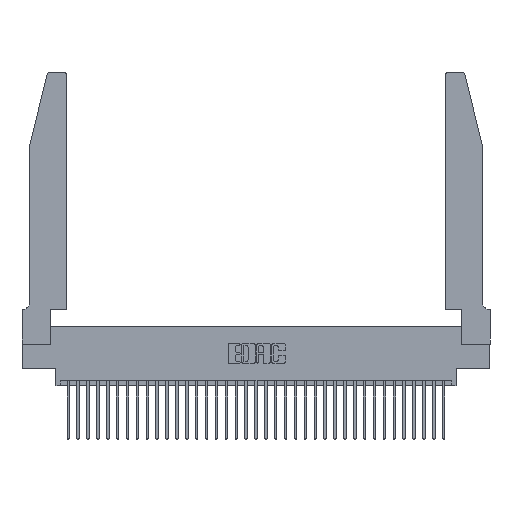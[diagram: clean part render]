
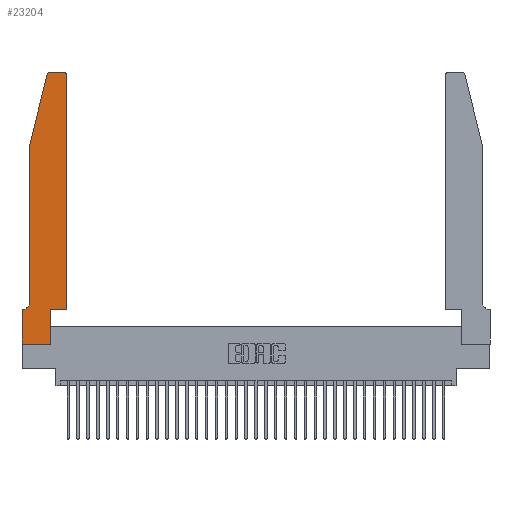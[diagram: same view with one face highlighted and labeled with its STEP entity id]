
A CAD part, top view. The second image highlights one B-rep face of the part: STEP entity #23204.
In plain terms, the highlighted planar face has unit normal (0, 0, 1).
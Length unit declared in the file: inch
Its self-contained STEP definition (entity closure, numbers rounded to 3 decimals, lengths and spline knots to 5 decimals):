
#298 = VECTOR ( 'NONE', #17683, 39.37008 ) ;
#578 = CIRCLE ( 'NONE', #31965, 0.07 ) ;
#1202 = DIRECTION ( 'NONE',  ( 0., 0., -1. ) ) ;
#1288 = VECTOR ( 'NONE', #32360, 39.37008 ) ;
#2203 = CARTESIAN_POINT ( 'NONE',  ( 0.0755, 2., 0.37 ) ) ;
#2274 = ORIENTED_EDGE ( 'NONE', *, *, #16135, .T. ) ;
#2450 = DIRECTION ( 'NONE',  ( -1., 0., 0. ) ) ;
#2820 = LINE ( 'NONE', #4468, #11868 ) ;
#3129 = ORIENTED_EDGE ( 'NONE', *, *, #24336, .T. ) ;
#3599 = CARTESIAN_POINT ( 'NONE',  ( 0., 0.35, 0.37 ) ) ;
#3640 = FACE_OUTER_BOUND ( 'NONE', #35420, .T. ) ;
#3865 = EDGE_CURVE ( 'NONE', #8779, #29767, #17887, .T. ) ;
#4079 = CARTESIAN_POINT ( 'NONE',  ( 0.4205, 2.75, 0.37 ) ) ;
#4468 = CARTESIAN_POINT ( 'NONE',  ( 0.0755, 2., 0.37 ) ) ;
#4948 = CARTESIAN_POINT ( 'NONE',  ( 0., 0., 0.37 ) ) ;
#5295 = ORIENTED_EDGE ( 'NONE', *, *, #23251, .T. ) ;
#5434 = DIRECTION ( 'NONE',  ( 0., -1., 0. ) ) ;
#6022 = CARTESIAN_POINT ( 'NONE',  ( 0., 0., 0.37 ) ) ;
#6300 = CARTESIAN_POINT ( 'NONE',  ( 0.2865, 0.35, 0.37 ) ) ;
#6398 = DIRECTION ( 'NONE',  ( 1., 0., 0. ) ) ;
#6543 = CARTESIAN_POINT ( 'NONE',  ( 0.4505, 0.35, 0.37 ) ) ;
#6659 = CARTESIAN_POINT ( 'NONE',  ( 0.2865, 0., 0.37 ) ) ;
#8052 = LINE ( 'NONE', #30765, #28008 ) ;
#8553 = EDGE_CURVE ( 'NONE', #35627, #26070, #19474, .T. ) ;
#8731 = EDGE_CURVE ( 'NONE', #12266, #22582, #26836, .T. ) ;
#8779 = VERTEX_POINT ( 'NONE', #23509 ) ;
#9349 = DIRECTION ( 'NONE',  ( 1., 0., 0. ) ) ;
#9463 = DIRECTION ( 'NONE',  ( 0., 0., 1. ) ) ;
#10051 = CARTESIAN_POINT ( 'NONE',  ( 0.284, 2.75, 0.37 ) ) ;
#10650 = LINE ( 'NONE', #14757, #29789 ) ;
#11107 = ORIENTED_EDGE ( 'NONE', *, *, #34659, .T. ) ;
#11378 = ORIENTED_EDGE ( 'NONE', *, *, #29390, .T. ) ;
#11567 = LINE ( 'NONE', #6543, #32030 ) ;
#11868 = VECTOR ( 'NONE', #23905, 39.37008 ) ;
#12096 = CARTESIAN_POINT ( 'NONE',  ( 0.0055, 0.42, 0.37 ) ) ;
#12266 = VERTEX_POINT ( 'NONE', #25598 ) ;
#12631 = CARTESIAN_POINT ( 'NONE',  ( 0.0755, 0.35, 0.37 ) ) ;
#13081 = CARTESIAN_POINT ( 'NONE',  ( 0.4505, 2.72, 0.37 ) ) ;
#13513 = CARTESIAN_POINT ( 'NONE',  ( 0.0755, 0.42, 0.37 ) ) ;
#13753 = VECTOR ( 'NONE', #2450, 39.37008 ) ;
#14757 = CARTESIAN_POINT ( 'NONE',  ( 0.2605, 2.75, 0.37 ) ) ;
#14795 = VERTEX_POINT ( 'NONE', #18711 ) ;
#14835 = DIRECTION ( 'NONE',  ( -1., 0., 0. ) ) ;
#15257 = VERTEX_POINT ( 'NONE', #10051 ) ;
#15481 = CARTESIAN_POINT ( 'NONE',  ( 0.4505, 0.35, 0.37 ) ) ;
#15888 = CARTESIAN_POINT ( 'NONE',  ( 0.4205, 2.72, 0.37 ) ) ;
#16135 = EDGE_CURVE ( 'NONE', #22582, #33917, #578, .T. ) ;
#16270 = LINE ( 'NONE', #17220, #22320 ) ;
#16754 = LINE ( 'NONE', #12631, #13753 ) ;
#17220 = CARTESIAN_POINT ( 'NONE',  ( 0.2865, 0.35, 0.37 ) ) ;
#17295 = ORIENTED_EDGE ( 'NONE', *, *, #21621, .T. ) ;
#17437 = PLANE ( 'NONE',  #19689 ) ;
#17547 = AXIS2_PLACEMENT_3D ( 'NONE', #23192, #9463, #9349 ) ;
#17683 = DIRECTION ( 'NONE',  ( 0., -1., 0. ) ) ;
#17887 = LINE ( 'NONE', #6022, #33146 ) ;
#18711 = CARTESIAN_POINT ( 'NONE',  ( 0.25487, 2.72718, 0.37 ) ) ;
#19187 = VERTEX_POINT ( 'NONE', #6659 ) ;
#19474 = CIRCLE ( 'NONE', #28625, 0.03 ) ;
#19689 = AXIS2_PLACEMENT_3D ( 'NONE', #3599, #23043, #6398 ) ;
#20548 = VERTEX_POINT ( 'NONE', #6300 ) ;
#21621 = EDGE_CURVE ( 'NONE', #15257, #14795, #30366, .T. ) ;
#21724 = DIRECTION ( 'NONE',  ( 0., 0., 1. ) ) ;
#22168 = CARTESIAN_POINT ( 'NONE',  ( 0.0055, 0.35, 0.37 ) ) ;
#22320 = VECTOR ( 'NONE', #33981, 39.37008 ) ;
#22582 = VERTEX_POINT ( 'NONE', #13513 ) ;
#22817 = EDGE_CURVE ( 'NONE', #33917, #8779, #16754, .T. ) ;
#23043 = DIRECTION ( 'NONE',  ( 0., 0., 1. ) ) ;
#23192 = CARTESIAN_POINT ( 'NONE',  ( 0.284, 2.72, 0.37 ) ) ;
#23204 = ADVANCED_FACE ( 'NONE', ( #3640 ), #17437, .T. ) ;
#23251 = EDGE_CURVE ( 'NONE', #14795, #12266, #2820, .T. ) ;
#23360 = ORIENTED_EDGE ( 'NONE', *, *, #8731, .T. ) ;
#23509 = CARTESIAN_POINT ( 'NONE',  ( 0., 0.35, 0.37 ) ) ;
#23905 = DIRECTION ( 'NONE',  ( -0.239, -0.971, 0. ) ) ;
#24336 = EDGE_CURVE ( 'NONE', #29767, #19187, #8052, .T. ) ;
#24509 = ORIENTED_EDGE ( 'NONE', *, *, #8553, .T. ) ;
#25598 = CARTESIAN_POINT ( 'NONE',  ( 0.0755, 2., 0.37 ) ) ;
#25603 = ORIENTED_EDGE ( 'NONE', *, *, #22817, .T. ) ;
#26070 = VERTEX_POINT ( 'NONE', #4079 ) ;
#26489 = LINE ( 'NONE', #15481, #1288 ) ;
#26836 = LINE ( 'NONE', #2203, #298 ) ;
#26852 = EDGE_CURVE ( 'NONE', #20548, #34391, #26489, .T. ) ;
#27296 = DIRECTION ( 'NONE',  ( 1., 0., 0. ) ) ;
#28008 = VECTOR ( 'NONE', #35088, 39.37008 ) ;
#28625 = AXIS2_PLACEMENT_3D ( 'NONE', #15888, #21724, #27296 ) ;
#28869 = DIRECTION ( 'NONE',  ( 0., 1., 0. ) ) ;
#29039 = ORIENTED_EDGE ( 'NONE', *, *, #32875, .T. ) ;
#29390 = EDGE_CURVE ( 'NONE', #26070, #15257, #10650, .T. ) ;
#29767 = VERTEX_POINT ( 'NONE', #4948 ) ;
#29789 = VECTOR ( 'NONE', #34173, 39.37008 ) ;
#30366 = CIRCLE ( 'NONE', #17547, 0.03 ) ;
#30719 = ORIENTED_EDGE ( 'NONE', *, *, #26852, .T. ) ;
#30765 = CARTESIAN_POINT ( 'NONE',  ( 0., 0., 0.37 ) ) ;
#31965 = AXIS2_PLACEMENT_3D ( 'NONE', #12096, #1202, #14835 ) ;
#32030 = VECTOR ( 'NONE', #28869, 39.37008 ) ;
#32360 = DIRECTION ( 'NONE',  ( 1., 0., 0. ) ) ;
#32875 = EDGE_CURVE ( 'NONE', #34391, #35627, #11567, .T. ) ;
#32958 = CARTESIAN_POINT ( 'NONE',  ( 0.4505, 0.35, 0.37 ) ) ;
#33146 = VECTOR ( 'NONE', #5434, 39.37008 ) ;
#33783 = ORIENTED_EDGE ( 'NONE', *, *, #3865, .T. ) ;
#33917 = VERTEX_POINT ( 'NONE', #22168 ) ;
#33981 = DIRECTION ( 'NONE',  ( 0., 1., 0. ) ) ;
#34173 = DIRECTION ( 'NONE',  ( -1., 0., 0. ) ) ;
#34391 = VERTEX_POINT ( 'NONE', #32958 ) ;
#34659 = EDGE_CURVE ( 'NONE', #19187, #20548, #16270, .T. ) ;
#35088 = DIRECTION ( 'NONE',  ( 1., 0., 0. ) ) ;
#35420 = EDGE_LOOP ( 'NONE', ( #11378, #17295, #5295, #23360, #2274, #25603, #33783, #3129, #11107, #30719, #29039, #24509 ) ) ;
#35627 = VERTEX_POINT ( 'NONE', #13081 ) ;
